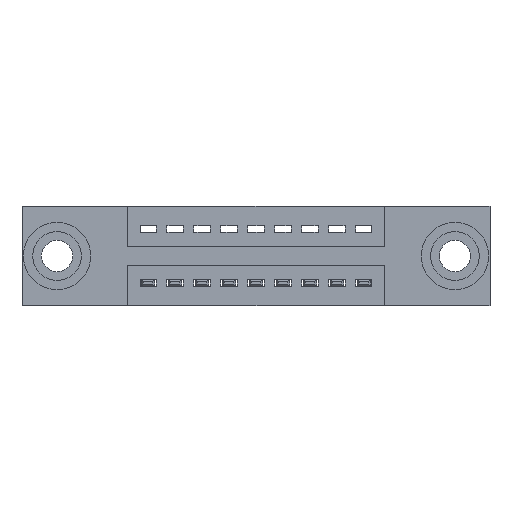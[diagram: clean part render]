
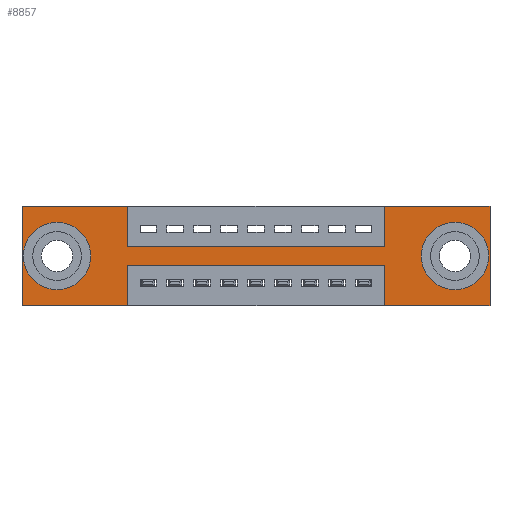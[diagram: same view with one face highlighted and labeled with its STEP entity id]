
A CAD part, front view. The second image highlights one B-rep face of the part: STEP entity #8857.
In plain terms, the highlighted planar face has unit normal (0, -1, 0).
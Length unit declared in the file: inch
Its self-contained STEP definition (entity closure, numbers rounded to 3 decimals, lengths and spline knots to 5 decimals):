
#127 = VECTOR ( 'NONE', #9878, 39.37008 ) ;
#172 = DIRECTION ( 'NONE',  ( 0., 0., 1. ) ) ;
#173 = FACE_OUTER_BOUND ( 'NONE', #8166, .T. ) ;
#182 = ORIENTED_EDGE ( 'NONE', *, *, #4278, .T. ) ;
#224 = VERTEX_POINT ( 'NONE', #727 ) ;
#415 = AXIS2_PLACEMENT_3D ( 'NONE', #486, #5244, #8858 ) ;
#440 = VERTEX_POINT ( 'NONE', #9192 ) ;
#486 = CARTESIAN_POINT ( 'NONE',  ( 1.605, 0., -0.185 ) ) ;
#514 = ORIENTED_EDGE ( 'NONE', *, *, #10766, .F. ) ;
#584 = VECTOR ( 'NONE', #10078, 39.37008 ) ;
#667 = CARTESIAN_POINT ( 'NONE',  ( 0.13, 0., -0.263 ) ) ;
#723 = FACE_BOUND ( 'NONE', #6301, .T. ) ;
#727 = CARTESIAN_POINT ( 'NONE',  ( 0.3925, 0., -0.22 ) ) ;
#826 = EDGE_CURVE ( 'NONE', #10321, #3474, #11087, .T. ) ;
#829 = DIRECTION ( 'NONE',  ( 0., 0., 1. ) ) ;
#831 = VERTEX_POINT ( 'NONE', #667 ) ;
#852 = VERTEX_POINT ( 'NONE', #2326 ) ;
#1034 = CARTESIAN_POINT ( 'NONE',  ( 0.3925, 0., -0.22 ) ) ;
#1035 = ORIENTED_EDGE ( 'NONE', *, *, #7696, .F. ) ;
#1289 = AXIS2_PLACEMENT_3D ( 'NONE', #1831, #11577, #6084 ) ;
#1499 = CARTESIAN_POINT ( 'NONE',  ( 1.3425, 0., 0. ) ) ;
#1630 = CARTESIAN_POINT ( 'NONE',  ( 1.735, 0., 0. ) ) ;
#1661 = AXIS2_PLACEMENT_3D ( 'NONE', #3862, #8366, #172 ) ;
#1720 = ORIENTED_EDGE ( 'NONE', *, *, #2840, .F. ) ;
#1831 = CARTESIAN_POINT ( 'NONE',  ( 1.605, 0., -0.185 ) ) ;
#1903 = VERTEX_POINT ( 'NONE', #1499 ) ;
#2326 = CARTESIAN_POINT ( 'NONE',  ( 1.3425, 0., -0.15 ) ) ;
#2351 = LINE ( 'NONE', #4593, #2513 ) ;
#2354 = VECTOR ( 'NONE', #9186, 39.37008 ) ;
#2439 = CIRCLE ( 'NONE', #1661, 0.078 ) ;
#2513 = VECTOR ( 'NONE', #5459, 39.37008 ) ;
#2585 = CARTESIAN_POINT ( 'NONE',  ( 1.605, 0., -0.263 ) ) ;
#2597 = ORIENTED_EDGE ( 'NONE', *, *, #4333, .T. ) ;
#2721 = VERTEX_POINT ( 'NONE', #11057 ) ;
#2765 = EDGE_CURVE ( 'NONE', #8901, #224, #8233, .T. ) ;
#2789 = EDGE_CURVE ( 'NONE', #852, #1903, #5547, .T. ) ;
#2840 = EDGE_CURVE ( 'NONE', #224, #7140, #6939, .T. ) ;
#2972 = ORIENTED_EDGE ( 'NONE', *, *, #10361, .F. ) ;
#3010 = CARTESIAN_POINT ( 'NONE',  ( 1.3425, 0., -0.37 ) ) ;
#3102 = AXIS2_PLACEMENT_3D ( 'NONE', #6251, #5354, #10689 ) ;
#3247 = EDGE_CURVE ( 'NONE', #11298, #10321, #5808, .T. ) ;
#3269 = VECTOR ( 'NONE', #4405, 39.37008 ) ;
#3312 = CARTESIAN_POINT ( 'NONE',  ( 0.3925, 0., 0. ) ) ;
#3365 = DIRECTION ( 'NONE',  ( -1., 0., 0. ) ) ;
#3474 = VERTEX_POINT ( 'NONE', #3010 ) ;
#3670 = LINE ( 'NONE', #9837, #127 ) ;
#3690 = ORIENTED_EDGE ( 'NONE', *, *, #3247, .F. ) ;
#3703 = ORIENTED_EDGE ( 'NONE', *, *, #2789, .F. ) ;
#3838 = AXIS2_PLACEMENT_3D ( 'NONE', #9714, #10656, #829 ) ;
#3862 = CARTESIAN_POINT ( 'NONE',  ( 0.13, 0., -0.185 ) ) ;
#3954 = CARTESIAN_POINT ( 'NONE',  ( 0., 0., 0. ) ) ;
#4242 = EDGE_LOOP ( 'NONE', ( #6870, #2597 ) ) ;
#4264 = EDGE_CURVE ( 'NONE', #7586, #852, #7346, .T. ) ;
#4278 = EDGE_CURVE ( 'NONE', #2721, #4319, #4534, .T. ) ;
#4319 = VERTEX_POINT ( 'NONE', #2585 ) ;
#4333 = EDGE_CURVE ( 'NONE', #831, #440, #7481, .T. ) ;
#4405 = DIRECTION ( 'NONE',  ( 0., 0., -1. ) ) ;
#4534 = CIRCLE ( 'NONE', #415, 0.078 ) ;
#4562 = VECTOR ( 'NONE', #5709, 39.37008 ) ;
#4593 = CARTESIAN_POINT ( 'NONE',  ( 0., 0., -0.37 ) ) ;
#4771 = VECTOR ( 'NONE', #3365, 39.37008 ) ;
#5066 = LINE ( 'NONE', #7336, #2354 ) ;
#5219 = EDGE_CURVE ( 'NONE', #7140, #8594, #2351, .T. ) ;
#5244 = DIRECTION ( 'NONE',  ( 0., 1., 0. ) ) ;
#5312 = VERTEX_POINT ( 'NONE', #9276 ) ;
#5354 = DIRECTION ( 'NONE',  ( 0., -1., 0. ) ) ;
#5459 = DIRECTION ( 'NONE',  ( -1., 0., 0. ) ) ;
#5547 = LINE ( 'NONE', #5638, #584 ) ;
#5638 = CARTESIAN_POINT ( 'NONE',  ( 1.3425, 0., 0. ) ) ;
#5643 = EDGE_CURVE ( 'NONE', #9528, #7586, #9007, .T. ) ;
#5684 = ORIENTED_EDGE ( 'NONE', *, *, #4264, .F. ) ;
#5709 = DIRECTION ( 'NONE',  ( 0., 0., -1. ) ) ;
#5790 = EDGE_CURVE ( 'NONE', #5312, #9528, #5066, .T. ) ;
#5808 = LINE ( 'NONE', #1630, #3269 ) ;
#5935 = ORIENTED_EDGE ( 'NONE', *, *, #5219, .F. ) ;
#6027 = VECTOR ( 'NONE', #8918, 39.37008 ) ;
#6084 = DIRECTION ( 'NONE',  ( 0., 0., -1. ) ) ;
#6089 = CARTESIAN_POINT ( 'NONE',  ( 0.3925, 0., -0.37 ) ) ;
#6251 = CARTESIAN_POINT ( 'NONE',  ( 0., 0., -0.37 ) ) ;
#6301 = EDGE_LOOP ( 'NONE', ( #182, #10987 ) ) ;
#6375 = VECTOR ( 'NONE', #8333, 39.37008 ) ;
#6732 = CARTESIAN_POINT ( 'NONE',  ( 0.3925, 0., -0.37 ) ) ;
#6802 = CARTESIAN_POINT ( 'NONE',  ( 0.3925, 0., -0.15 ) ) ;
#6870 = ORIENTED_EDGE ( 'NONE', *, *, #8417, .T. ) ;
#6939 = LINE ( 'NONE', #6732, #4562 ) ;
#7029 = DIRECTION ( 'NONE',  ( 0., 0., 1. ) ) ;
#7140 = VERTEX_POINT ( 'NONE', #6089 ) ;
#7336 = CARTESIAN_POINT ( 'NONE',  ( 0., 0., 0. ) ) ;
#7346 = LINE ( 'NONE', #6802, #8895 ) ;
#7409 = VECTOR ( 'NONE', #7029, 39.37008 ) ;
#7481 = CIRCLE ( 'NONE', #3838, 0.078 ) ;
#7540 = DIRECTION ( 'NONE',  ( 1., 0., 0. ) ) ;
#7586 = VERTEX_POINT ( 'NONE', #10153 ) ;
#7626 = CARTESIAN_POINT ( 'NONE',  ( 0.3925, 0., 0. ) ) ;
#7696 = EDGE_CURVE ( 'NONE', #8594, #5312, #11488, .T. ) ;
#7793 = CARTESIAN_POINT ( 'NONE',  ( 0., 0., -0.37 ) ) ;
#8166 = EDGE_LOOP ( 'NONE', ( #1720, #10360, #2972, #8972, #3690, #514, #3703, #5684, #11107, #9647, #1035, #5935 ) ) ;
#8233 = LINE ( 'NONE', #1034, #6375 ) ;
#8333 = DIRECTION ( 'NONE',  ( -1., 0., 0. ) ) ;
#8366 = DIRECTION ( 'NONE',  ( 0., 1., 0. ) ) ;
#8417 = EDGE_CURVE ( 'NONE', #440, #831, #2439, .T. ) ;
#8594 = VERTEX_POINT ( 'NONE', #10146 ) ;
#8857 = ADVANCED_FACE ( 'NONE', ( #723, #10051, #173 ), #9862, .T. ) ;
#8858 = DIRECTION ( 'NONE',  ( 0., 0., -1. ) ) ;
#8895 = VECTOR ( 'NONE', #10585, 39.37008 ) ;
#8901 = VERTEX_POINT ( 'NONE', #9902 ) ;
#8918 = DIRECTION ( 'NONE',  ( 0., 0., -1. ) ) ;
#8972 = ORIENTED_EDGE ( 'NONE', *, *, #826, .F. ) ;
#9007 = LINE ( 'NONE', #3312, #6027 ) ;
#9028 = LINE ( 'NONE', #3954, #10281 ) ;
#9186 = DIRECTION ( 'NONE',  ( 1., 0., 0. ) ) ;
#9192 = CARTESIAN_POINT ( 'NONE',  ( 0.13, 0., -0.107 ) ) ;
#9276 = CARTESIAN_POINT ( 'NONE',  ( 0., 0., 0. ) ) ;
#9323 = CIRCLE ( 'NONE', #1289, 0.078 ) ;
#9528 = VERTEX_POINT ( 'NONE', #7626 ) ;
#9647 = ORIENTED_EDGE ( 'NONE', *, *, #5790, .F. ) ;
#9714 = CARTESIAN_POINT ( 'NONE',  ( 0.13, 0., -0.185 ) ) ;
#9837 = CARTESIAN_POINT ( 'NONE',  ( 1.3425, 0., -0.37 ) ) ;
#9862 = PLANE ( 'NONE',  #3102 ) ;
#9878 = DIRECTION ( 'NONE',  ( 0., 0., 1. ) ) ;
#9902 = CARTESIAN_POINT ( 'NONE',  ( 1.3425, 0., -0.22 ) ) ;
#10045 = CARTESIAN_POINT ( 'NONE',  ( 1.735, 0., 0. ) ) ;
#10051 = FACE_BOUND ( 'NONE', #4242, .T. ) ;
#10078 = DIRECTION ( 'NONE',  ( 0., 0., 1. ) ) ;
#10146 = CARTESIAN_POINT ( 'NONE',  ( 0., 0., -0.37 ) ) ;
#10153 = CARTESIAN_POINT ( 'NONE',  ( 0.3925, 0., -0.15 ) ) ;
#10275 = EDGE_CURVE ( 'NONE', #4319, #2721, #9323, .T. ) ;
#10281 = VECTOR ( 'NONE', #7540, 39.37008 ) ;
#10321 = VERTEX_POINT ( 'NONE', #10809 ) ;
#10360 = ORIENTED_EDGE ( 'NONE', *, *, #2765, .F. ) ;
#10361 = EDGE_CURVE ( 'NONE', #3474, #8901, #3670, .T. ) ;
#10585 = DIRECTION ( 'NONE',  ( 1., 0., 0. ) ) ;
#10656 = DIRECTION ( 'NONE',  ( 0., 1., 0. ) ) ;
#10689 = DIRECTION ( 'NONE',  ( 0., 0., -1. ) ) ;
#10766 = EDGE_CURVE ( 'NONE', #1903, #11298, #9028, .T. ) ;
#10809 = CARTESIAN_POINT ( 'NONE',  ( 1.735, 0., -0.37 ) ) ;
#10987 = ORIENTED_EDGE ( 'NONE', *, *, #10275, .T. ) ;
#11057 = CARTESIAN_POINT ( 'NONE',  ( 1.605, 0., -0.107 ) ) ;
#11087 = LINE ( 'NONE', #7793, #4771 ) ;
#11107 = ORIENTED_EDGE ( 'NONE', *, *, #5643, .F. ) ;
#11298 = VERTEX_POINT ( 'NONE', #10045 ) ;
#11488 = LINE ( 'NONE', #11533, #7409 ) ;
#11533 = CARTESIAN_POINT ( 'NONE',  ( 0., 0., 0. ) ) ;
#11577 = DIRECTION ( 'NONE',  ( 0., 1., 0. ) ) ;
